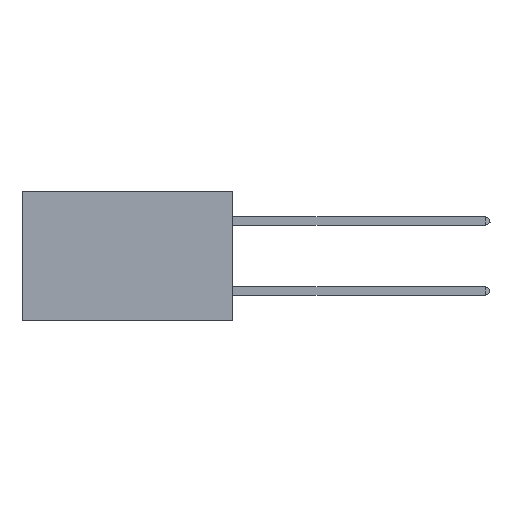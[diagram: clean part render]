
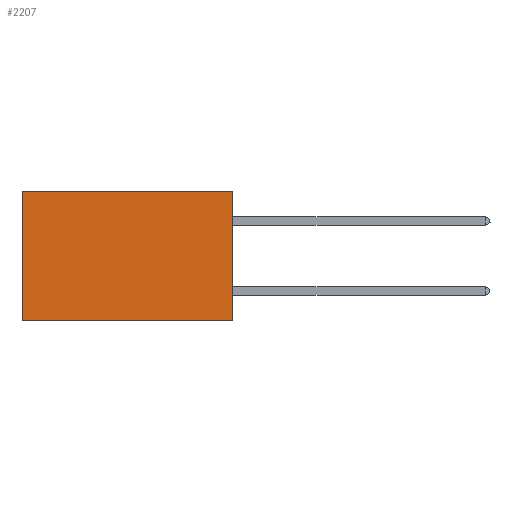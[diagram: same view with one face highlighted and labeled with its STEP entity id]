
A CAD part, left-side view. The second image highlights one B-rep face of the part: STEP entity #2207.
In plain terms, the highlighted planar face has unit normal (-1, 0, 0).
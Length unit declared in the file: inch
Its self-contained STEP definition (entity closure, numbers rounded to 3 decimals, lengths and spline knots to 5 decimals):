
#612 = VERTEX_POINT ( 'NONE', #15763 ) ;
#948 = VECTOR ( 'NONE', #5707, 39.37008 ) ;
#1089 = DIRECTION ( 'NONE',  ( 0., 0., -1. ) ) ;
#1348 = FACE_OUTER_BOUND ( 'NONE', #9976, .T. ) ;
#1885 = EDGE_CURVE ( 'NONE', #612, #8114, #9017, .T. ) ;
#2207 = ADVANCED_FACE ( 'NONE', ( #1348 ), #5335, .F. ) ;
#2305 = LINE ( 'NONE', #19423, #21659 ) ;
#3776 = CARTESIAN_POINT ( 'NONE',  ( 0.2875, 0., -0.37 ) ) ;
#3814 = ORIENTED_EDGE ( 'NONE', *, *, #24223, .T. ) ;
#4027 = EDGE_CURVE ( 'NONE', #22272, #21797, #5695, .T. ) ;
#4755 = AXIS2_PLACEMENT_3D ( 'NONE', #10983, #11517, #7509 ) ;
#5335 = PLANE ( 'NONE',  #4755 ) ;
#5695 = LINE ( 'NONE', #7642, #948 ) ;
#5707 = DIRECTION ( 'NONE',  ( 0., 0., -1. ) ) ;
#6082 = DIRECTION ( 'NONE',  ( 0., 1., 0. ) ) ;
#6101 = CARTESIAN_POINT ( 'NONE',  ( 0.2875, 0., 0. ) ) ;
#7058 = CARTESIAN_POINT ( 'NONE',  ( 0.2875, 0., -0.37 ) ) ;
#7509 = DIRECTION ( 'NONE',  ( 0., 0., -1. ) ) ;
#7586 = DIRECTION ( 'NONE',  ( 0., 1., 0. ) ) ;
#7642 = CARTESIAN_POINT ( 'NONE',  ( 0.2875, 0., 0. ) ) ;
#8114 = VERTEX_POINT ( 'NONE', #19932 ) ;
#9017 = LINE ( 'NONE', #18020, #10795 ) ;
#9976 = EDGE_LOOP ( 'NONE', ( #12449, #15255, #10894, #3814 ) ) ;
#10450 = VECTOR ( 'NONE', #7586, 39.37008 ) ;
#10795 = VECTOR ( 'NONE', #1089, 39.37008 ) ;
#10894 = ORIENTED_EDGE ( 'NONE', *, *, #4027, .F. ) ;
#10983 = CARTESIAN_POINT ( 'NONE',  ( 0.2875, 0., 0. ) ) ;
#11172 = EDGE_CURVE ( 'NONE', #21797, #8114, #17210, .T. ) ;
#11517 = DIRECTION ( 'NONE',  ( 1., 0., 0. ) ) ;
#12449 = ORIENTED_EDGE ( 'NONE', *, *, #1885, .T. ) ;
#15255 = ORIENTED_EDGE ( 'NONE', *, *, #11172, .F. ) ;
#15763 = CARTESIAN_POINT ( 'NONE',  ( 0.2875, 0.6, 0. ) ) ;
#17210 = LINE ( 'NONE', #3776, #10450 ) ;
#18020 = CARTESIAN_POINT ( 'NONE',  ( 0.2875, 0.6, 0. ) ) ;
#19423 = CARTESIAN_POINT ( 'NONE',  ( 0.2875, 0., 0. ) ) ;
#19932 = CARTESIAN_POINT ( 'NONE',  ( 0.2875, 0.6, -0.37 ) ) ;
#21659 = VECTOR ( 'NONE', #6082, 39.37008 ) ;
#21797 = VERTEX_POINT ( 'NONE', #7058 ) ;
#22272 = VERTEX_POINT ( 'NONE', #6101 ) ;
#24223 = EDGE_CURVE ( 'NONE', #22272, #612, #2305, .T. ) ;
